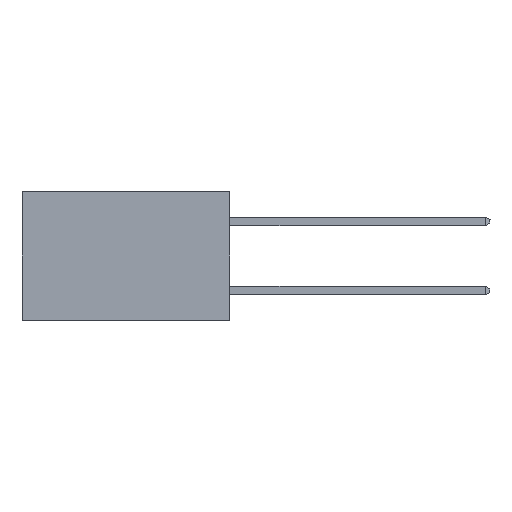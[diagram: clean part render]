
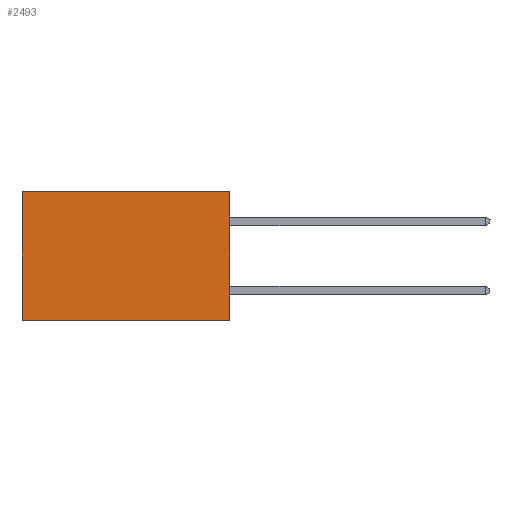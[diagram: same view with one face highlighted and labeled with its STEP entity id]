
A CAD part, left-side view. The second image highlights one B-rep face of the part: STEP entity #2493.
In plain terms, the highlighted planar face has unit normal (-1, 0, 0).
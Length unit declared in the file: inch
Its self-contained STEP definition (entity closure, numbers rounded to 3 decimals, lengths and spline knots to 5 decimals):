
#17 = DIRECTION ( 'NONE',  ( 0., 0., -1. ) ) ;
#1086 = ORIENTED_EDGE ( 'NONE', *, *, #6498, .F. ) ;
#2007 = VERTEX_POINT ( 'NONE', #20431 ) ;
#2052 = ORIENTED_EDGE ( 'NONE', *, *, #10995, .T. ) ;
#2493 = ADVANCED_FACE ( 'NONE', ( #9553 ), #14753, .F. ) ;
#3596 = CARTESIAN_POINT ( 'NONE',  ( 0.298, 0., 0. ) ) ;
#3835 = DIRECTION ( 'NONE',  ( 0., 0., -1. ) ) ;
#4761 = DIRECTION ( 'NONE',  ( 0., 1., 0. ) ) ;
#5700 = CARTESIAN_POINT ( 'NONE',  ( 0.298, 0., 0. ) ) ;
#6498 = EDGE_CURVE ( 'NONE', #2007, #19750, #20876, .T. ) ;
#6619 = VERTEX_POINT ( 'NONE', #18021 ) ;
#7124 = LINE ( 'NONE', #3596, #14673 ) ;
#8449 = CARTESIAN_POINT ( 'NONE',  ( 0.298, 0.6, 0. ) ) ;
#8794 = DIRECTION ( 'NONE',  ( 0., 1., 0. ) ) ;
#9327 = DIRECTION ( 'NONE',  ( 1., 0., 0. ) ) ;
#9553 = FACE_OUTER_BOUND ( 'NONE', #19534, .T. ) ;
#10348 = EDGE_CURVE ( 'NONE', #16076, #19750, #19596, .T. ) ;
#10377 = CARTESIAN_POINT ( 'NONE',  ( 0.298, 0.6, -0.37 ) ) ;
#10995 = EDGE_CURVE ( 'NONE', #6619, #16076, #20656, .T. ) ;
#11674 = ORIENTED_EDGE ( 'NONE', *, *, #10348, .T. ) ;
#11691 = VECTOR ( 'NONE', #4761, 39.37008 ) ;
#13635 = CARTESIAN_POINT ( 'NONE',  ( 0.298, 0., 0. ) ) ;
#14523 = CARTESIAN_POINT ( 'NONE',  ( 0.298, 0.6, 0. ) ) ;
#14673 = VECTOR ( 'NONE', #17, 39.37008 ) ;
#14753 = PLANE ( 'NONE',  #19244 ) ;
#14889 = ORIENTED_EDGE ( 'NONE', *, *, #20022, .F. ) ;
#15849 = CARTESIAN_POINT ( 'NONE',  ( 0.298, 0., -0.37 ) ) ;
#16076 = VERTEX_POINT ( 'NONE', #14523 ) ;
#18021 = CARTESIAN_POINT ( 'NONE',  ( 0.298, 0., 0. ) ) ;
#19244 = AXIS2_PLACEMENT_3D ( 'NONE', #5700, #9327, #3835 ) ;
#19534 = EDGE_LOOP ( 'NONE', ( #11674, #1086, #14889, #2052 ) ) ;
#19596 = LINE ( 'NONE', #8449, #19871 ) ;
#19750 = VERTEX_POINT ( 'NONE', #10377 ) ;
#19871 = VECTOR ( 'NONE', #20847, 39.37008 ) ;
#20022 = EDGE_CURVE ( 'NONE', #6619, #2007, #7124, .T. ) ;
#20431 = CARTESIAN_POINT ( 'NONE',  ( 0.298, 0., -0.37 ) ) ;
#20656 = LINE ( 'NONE', #13635, #11691 ) ;
#20847 = DIRECTION ( 'NONE',  ( 0., 0., -1. ) ) ;
#20876 = LINE ( 'NONE', #15849, #21167 ) ;
#21167 = VECTOR ( 'NONE', #8794, 39.37008 ) ;
